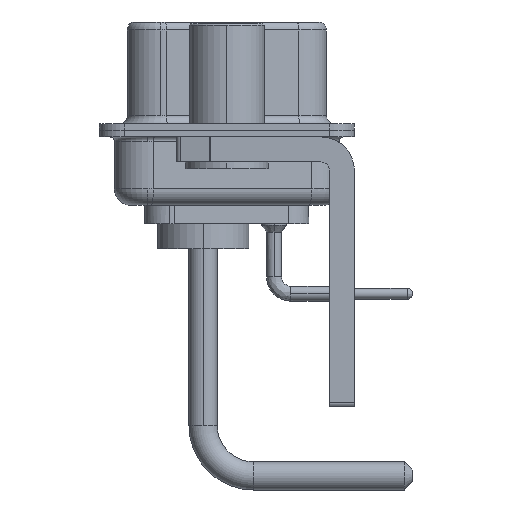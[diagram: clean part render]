
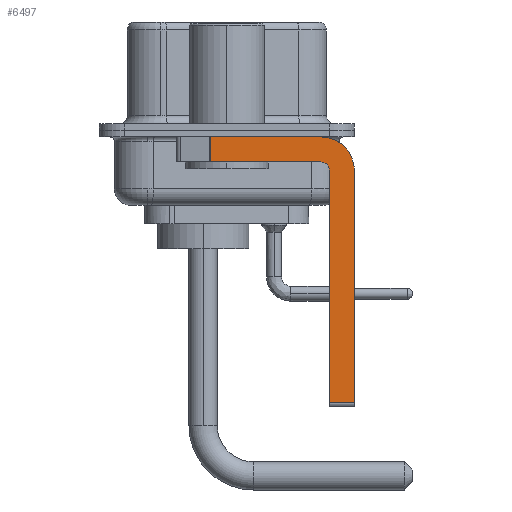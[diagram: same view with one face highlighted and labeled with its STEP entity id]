
A CAD part, left-side view. The second image highlights one B-rep face of the part: STEP entity #6497.
In plain terms, the highlighted planar face has unit normal (-1, 0, 0).
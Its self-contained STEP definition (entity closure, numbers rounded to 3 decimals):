
#425 = VERTEX_POINT ( 'NONE', #2460 ) ;
#582 = CARTESIAN_POINT ( 'NONE',  ( -2.9, 0.978, -0.4 ) ) ;
#980 = VERTEX_POINT ( 'NONE', #3085 ) ;
#1149 = DIRECTION ( 'NONE',  ( 0., 1., 0. ) ) ;
#1157 = CARTESIAN_POINT ( 'NONE',  ( -2.9, -6.15, -16.35 ) ) ;
#1585 = VERTEX_POINT ( 'NONE', #14086 ) ;
#2073 = CARTESIAN_POINT ( 'NONE',  ( -2.9, 0.978, -1.9 ) ) ;
#2285 = EDGE_CURVE ( 'NONE', #15462, #19807, #4536, .T. ) ;
#2460 = CARTESIAN_POINT ( 'NONE',  ( -2.9, -5.65, -1.9 ) ) ;
#2866 = FACE_OUTER_BOUND ( 'NONE', #5978, .T. ) ;
#3085 = CARTESIAN_POINT ( 'NONE',  ( -2.9, 0.978, -1.9 ) ) ;
#3229 = CIRCLE ( 'NONE', #18144, 2. ) ;
#4536 = LINE ( 'NONE', #12791, #26245 ) ;
#4652 = VERTEX_POINT ( 'NONE', #13134 ) ;
#4883 = DIRECTION ( 'NONE',  ( 0., 0., 1. ) ) ;
#5253 = ORIENTED_EDGE ( 'NONE', *, *, #16938, .T. ) ;
#5266 = PLANE ( 'NONE',  #15912 ) ;
#5297 = CARTESIAN_POINT ( 'NONE',  ( -2.9, -5.65, -1.9 ) ) ;
#5978 = EDGE_LOOP ( 'NONE', ( #18298, #5253, #7859, #22435, #17043, #8229, #21838, #16992 ) ) ;
#6095 = VECTOR ( 'NONE', #1149, 1000. ) ;
#6128 = EDGE_CURVE ( 'NONE', #425, #980, #15302, .T. ) ;
#6497 = ADVANCED_FACE ( 'NONE', ( #2866 ), #5266, .F. ) ;
#7635 = EDGE_CURVE ( 'NONE', #10309, #425, #11208, .T. ) ;
#7859 = ORIENTED_EDGE ( 'NONE', *, *, #6128, .F. ) ;
#8229 = ORIENTED_EDGE ( 'NONE', *, *, #2285, .T. ) ;
#10309 = VERTEX_POINT ( 'NONE', #22037 ) ;
#10437 = CARTESIAN_POINT ( 'NONE',  ( -2.9, -7.65, -16.35 ) ) ;
#11013 = EDGE_CURVE ( 'NONE', #15462, #10309, #19430, .T. ) ;
#11208 = CIRCLE ( 'NONE', #25713, 0.5 ) ;
#11490 = DIRECTION ( 'NONE',  ( 1., 0., 0. ) ) ;
#11494 = VERTEX_POINT ( 'NONE', #582 ) ;
#12427 = EDGE_CURVE ( 'NONE', #11494, #1585, #19316, .T. ) ;
#12791 = CARTESIAN_POINT ( 'NONE',  ( -2.9, -5.65, -16.35 ) ) ;
#12880 = LINE ( 'NONE', #21035, #22091 ) ;
#13000 = DIRECTION ( 'NONE',  ( 0., 0., 1. ) ) ;
#13134 = CARTESIAN_POINT ( 'NONE',  ( -2.9, -7.65, -2.4 ) ) ;
#13145 = DIRECTION ( 'NONE',  ( 0., 0., -1. ) ) ;
#13347 = DIRECTION ( 'NONE',  ( 0., 0., -1. ) ) ;
#13400 = DIRECTION ( 'NONE',  ( -1., 0., 0. ) ) ;
#13974 = LINE ( 'NONE', #2073, #17610 ) ;
#14086 = CARTESIAN_POINT ( 'NONE',  ( -2.9, -5.65, -0.4 ) ) ;
#15200 = DIRECTION ( 'NONE',  ( 0., -1., 0. ) ) ;
#15302 = LINE ( 'NONE', #5297, #6095 ) ;
#15462 = VERTEX_POINT ( 'NONE', #1157 ) ;
#15912 = AXIS2_PLACEMENT_3D ( 'NONE', #23181, #21288, #21422 ) ;
#16938 = EDGE_CURVE ( 'NONE', #11494, #980, #13974, .T. ) ;
#16992 = ORIENTED_EDGE ( 'NONE', *, *, #19482, .F. ) ;
#17043 = ORIENTED_EDGE ( 'NONE', *, *, #11013, .F. ) ;
#17610 = VECTOR ( 'NONE', #20235, 1000. ) ;
#18144 = AXIS2_PLACEMENT_3D ( 'NONE', #19628, #11490, #13347 ) ;
#18298 = ORIENTED_EDGE ( 'NONE', *, *, #12427, .F. ) ;
#19055 = CARTESIAN_POINT ( 'NONE',  ( -2.9, 3., -0.4 ) ) ;
#19316 = LINE ( 'NONE', #19055, #20338 ) ;
#19430 = LINE ( 'NONE', #21438, #21598 ) ;
#19482 = EDGE_CURVE ( 'NONE', #1585, #4652, #3229, .T. ) ;
#19552 = CARTESIAN_POINT ( 'NONE',  ( -2.9, -5.65, -2.4 ) ) ;
#19628 = CARTESIAN_POINT ( 'NONE',  ( -2.9, -5.65, -2.4 ) ) ;
#19807 = VERTEX_POINT ( 'NONE', #10437 ) ;
#20235 = DIRECTION ( 'NONE',  ( 0., 0., -1. ) ) ;
#20338 = VECTOR ( 'NONE', #23614, 1000. ) ;
#21035 = CARTESIAN_POINT ( 'NONE',  ( -2.9, -7.65, -2.4 ) ) ;
#21288 = DIRECTION ( 'NONE',  ( 1., 0., 0. ) ) ;
#21422 = DIRECTION ( 'NONE',  ( 0., 0., -1. ) ) ;
#21438 = CARTESIAN_POINT ( 'NONE',  ( -2.9, -6.15, -16.6 ) ) ;
#21598 = VECTOR ( 'NONE', #4883, 1000. ) ;
#21838 = ORIENTED_EDGE ( 'NONE', *, *, #22801, .F. ) ;
#22037 = CARTESIAN_POINT ( 'NONE',  ( -2.9, -6.15, -2.4 ) ) ;
#22091 = VECTOR ( 'NONE', #13145, 1000. ) ;
#22435 = ORIENTED_EDGE ( 'NONE', *, *, #7635, .F. ) ;
#22801 = EDGE_CURVE ( 'NONE', #4652, #19807, #12880, .T. ) ;
#23181 = CARTESIAN_POINT ( 'NONE',  ( -2.9, -5.65, -2.4 ) ) ;
#23614 = DIRECTION ( 'NONE',  ( 0., -1., 0. ) ) ;
#25713 = AXIS2_PLACEMENT_3D ( 'NONE', #19552, #13400, #13000 ) ;
#26245 = VECTOR ( 'NONE', #15200, 1000. ) ;
